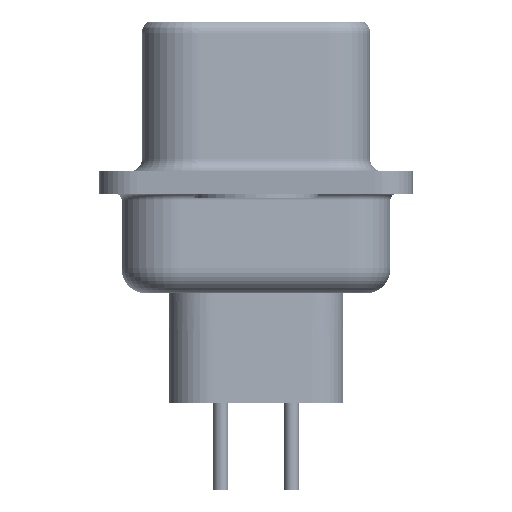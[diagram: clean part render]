
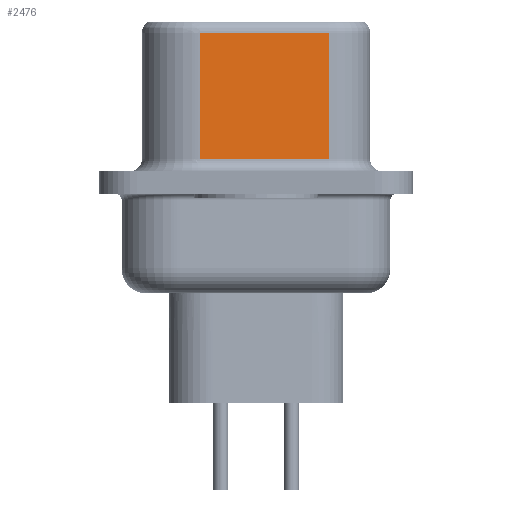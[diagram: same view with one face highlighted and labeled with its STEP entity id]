
A CAD part, left-side view. The second image highlights one B-rep face of the part: STEP entity #2476.
In plain terms, the highlighted planar face has unit normal (-0.985, -0.174, 0).
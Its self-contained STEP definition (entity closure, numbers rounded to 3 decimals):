
#36 = VERTEX_POINT ( 'NONE', #15219 ) ;
#606 = VERTEX_POINT ( 'NONE', #8920 ) ;
#2476 = ADVANCED_FACE ( 'NONE', ( #16258 ), #14075, .F. ) ;
#2733 = DIRECTION ( 'NONE',  ( 0., 0., -1. ) ) ;
#2894 = VECTOR ( 'NONE', #4367, 1000. ) ;
#4367 = DIRECTION ( 'NONE',  ( -0.174, 0.985, 0. ) ) ;
#5067 = LINE ( 'NONE', #9267, #25815 ) ;
#5661 = EDGE_LOOP ( 'NONE', ( #24764, #15207, #29186, #23519 ) ) ;
#5940 = VECTOR ( 'NONE', #2733, 1000. ) ;
#6481 = DIRECTION ( 'NONE',  ( 0.174, -0.985, 0. ) ) ;
#7536 = LINE ( 'NONE', #17006, #5940 ) ;
#7795 = AXIS2_PLACEMENT_3D ( 'NONE', #11599, #30553, #18729 ) ;
#8452 = LINE ( 'NONE', #17931, #2894 ) ;
#8920 = CARTESIAN_POINT ( 'NONE',  ( 4.58, -2.927, 0.95 ) ) ;
#9267 = CARTESIAN_POINT ( 'NONE',  ( 3.67, 2.233, 6.52 ) ) ;
#10745 = CARTESIAN_POINT ( 'NONE',  ( 3.67, 2.233, 6.02 ) ) ;
#11462 = DIRECTION ( 'NONE',  ( 0., 0., -1. ) ) ;
#11599 = CARTESIAN_POINT ( 'NONE',  ( 4.58, -2.927, 6.52 ) ) ;
#11687 = VERTEX_POINT ( 'NONE', #26654 ) ;
#11889 = CARTESIAN_POINT ( 'NONE',  ( 4.58, -2.927, 0.95 ) ) ;
#14075 = PLANE ( 'NONE',  #7795 ) ;
#15207 = ORIENTED_EDGE ( 'NONE', *, *, #15576, .T. ) ;
#15219 = CARTESIAN_POINT ( 'NONE',  ( 4.58, -2.927, 6.02 ) ) ;
#15576 = EDGE_CURVE ( 'NONE', #36, #21246, #8452, .T. ) ;
#16258 = FACE_OUTER_BOUND ( 'NONE', #5661, .T. ) ;
#17006 = CARTESIAN_POINT ( 'NONE',  ( 4.58, -2.927, 6.52 ) ) ;
#17931 = CARTESIAN_POINT ( 'NONE',  ( 4.58, -2.927, 6.02 ) ) ;
#18662 = EDGE_CURVE ( 'NONE', #21246, #11687, #5067, .T. ) ;
#18729 = DIRECTION ( 'NONE',  ( -0.174, 0.985, 0. ) ) ;
#21246 = VERTEX_POINT ( 'NONE', #10745 ) ;
#21366 = LINE ( 'NONE', #11889, #27031 ) ;
#23519 = ORIENTED_EDGE ( 'NONE', *, *, #23913, .T. ) ;
#23913 = EDGE_CURVE ( 'NONE', #11687, #606, #21366, .T. ) ;
#24764 = ORIENTED_EDGE ( 'NONE', *, *, #25390, .F. ) ;
#25390 = EDGE_CURVE ( 'NONE', #36, #606, #7536, .T. ) ;
#25815 = VECTOR ( 'NONE', #11462, 1000. ) ;
#26654 = CARTESIAN_POINT ( 'NONE',  ( 3.67, 2.233, 0.95 ) ) ;
#27031 = VECTOR ( 'NONE', #6481, 1000. ) ;
#29186 = ORIENTED_EDGE ( 'NONE', *, *, #18662, .T. ) ;
#30553 = DIRECTION ( 'NONE',  ( 0.985, 0.174, 0. ) ) ;
